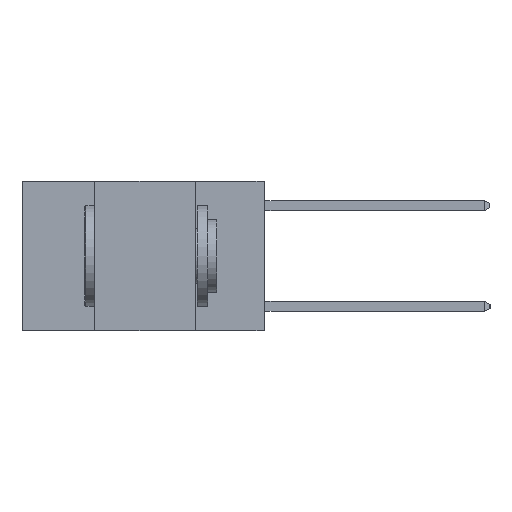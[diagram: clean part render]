
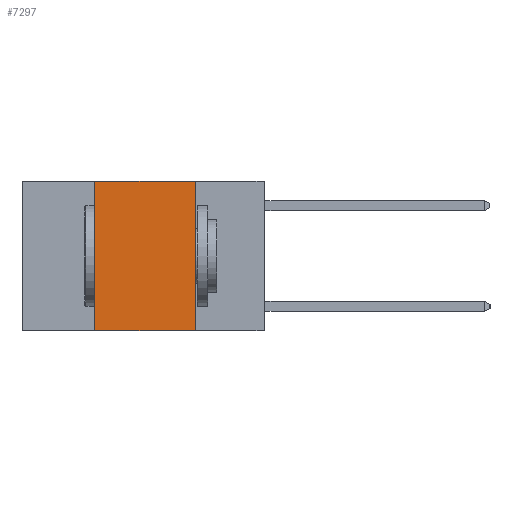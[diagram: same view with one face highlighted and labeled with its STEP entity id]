
A CAD part, left-side view. The second image highlights one B-rep face of the part: STEP entity #7297.
In plain terms, the highlighted planar face has unit normal (-1, 0, 0).
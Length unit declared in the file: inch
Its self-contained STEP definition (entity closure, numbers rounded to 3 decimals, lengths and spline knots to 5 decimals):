
#40 = LINE ( 'NONE', #1205, #2193 ) ;
#114 = VECTOR ( 'NONE', #2117, 39.37008 ) ;
#129 = FACE_OUTER_BOUND ( 'NONE', #1825, .T. ) ;
#133 = CARTESIAN_POINT ( 'NONE',  ( 0., 0.42, -0.37 ) ) ;
#190 = EDGE_CURVE ( 'NONE', #2527, #594, #2047, .T. ) ;
#250 = DIRECTION ( 'NONE',  ( 1., 0., 0. ) ) ;
#457 = DIRECTION ( 'NONE',  ( 0., 0., -1. ) ) ;
#594 = VERTEX_POINT ( 'NONE', #8746 ) ;
#670 = ORIENTED_EDGE ( 'NONE', *, *, #5775, .F. ) ;
#1190 = VECTOR ( 'NONE', #5643, 39.37008 ) ;
#1205 = CARTESIAN_POINT ( 'NONE',  ( 0., 0.17, 0. ) ) ;
#1695 = AXIS2_PLACEMENT_3D ( 'NONE', #7457, #250, #5326 ) ;
#1825 = EDGE_LOOP ( 'NONE', ( #8848, #4819, #670, #9320 ) ) ;
#2018 = VECTOR ( 'NONE', #4342, 39.37008 ) ;
#2047 = LINE ( 'NONE', #6140, #114 ) ;
#2117 = DIRECTION ( 'NONE',  ( 0., -1., 0. ) ) ;
#2193 = VECTOR ( 'NONE', #457, 39.37008 ) ;
#2511 = CARTESIAN_POINT ( 'NONE',  ( 0., 0.42, 0. ) ) ;
#2527 = VERTEX_POINT ( 'NONE', #133 ) ;
#3431 = VERTEX_POINT ( 'NONE', #8389 ) ;
#3641 = EDGE_CURVE ( 'NONE', #4888, #3431, #3922, .T. ) ;
#3922 = LINE ( 'NONE', #4390, #2018 ) ;
#4342 = DIRECTION ( 'NONE',  ( 0., -1., 0. ) ) ;
#4390 = CARTESIAN_POINT ( 'NONE',  ( 0., 0.6, 0. ) ) ;
#4582 = PLANE ( 'NONE',  #1695 ) ;
#4819 = ORIENTED_EDGE ( 'NONE', *, *, #3641, .F. ) ;
#4888 = VERTEX_POINT ( 'NONE', #2511 ) ;
#4898 = CARTESIAN_POINT ( 'NONE',  ( 0., 0.42, 0. ) ) ;
#5031 = LINE ( 'NONE', #4898, #1190 ) ;
#5326 = DIRECTION ( 'NONE',  ( 0., 0., -1. ) ) ;
#5643 = DIRECTION ( 'NONE',  ( 0., 0., 1. ) ) ;
#5775 = EDGE_CURVE ( 'NONE', #2527, #4888, #5031, .T. ) ;
#6140 = CARTESIAN_POINT ( 'NONE',  ( 0., 0.6, -0.37 ) ) ;
#6246 = EDGE_CURVE ( 'NONE', #3431, #594, #40, .T. ) ;
#7297 = ADVANCED_FACE ( 'NONE', ( #129 ), #4582, .F. ) ;
#7457 = CARTESIAN_POINT ( 'NONE',  ( 0., 0.6, 0. ) ) ;
#8389 = CARTESIAN_POINT ( 'NONE',  ( 0., 0.17, 0. ) ) ;
#8746 = CARTESIAN_POINT ( 'NONE',  ( 0., 0.17, -0.37 ) ) ;
#8848 = ORIENTED_EDGE ( 'NONE', *, *, #6246, .F. ) ;
#9320 = ORIENTED_EDGE ( 'NONE', *, *, #190, .T. ) ;
